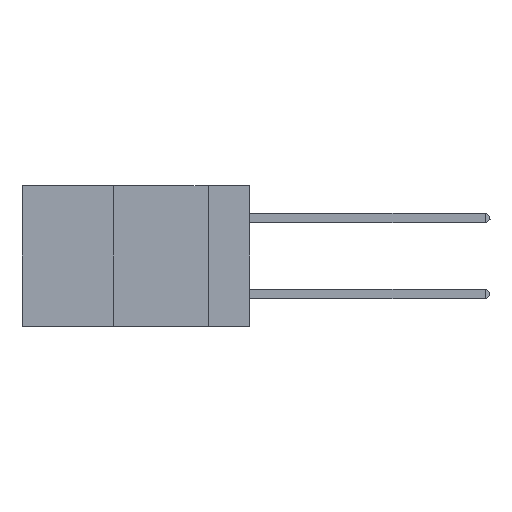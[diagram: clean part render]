
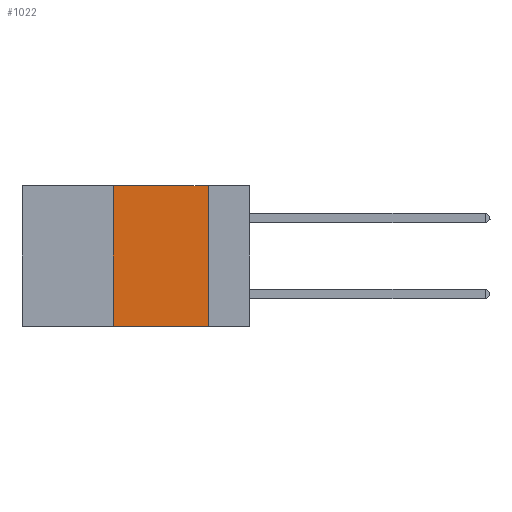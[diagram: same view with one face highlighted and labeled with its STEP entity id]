
A CAD part, left-side view. The second image highlights one B-rep face of the part: STEP entity #1022.
In plain terms, the highlighted planar face has unit normal (-1, 0, 0).
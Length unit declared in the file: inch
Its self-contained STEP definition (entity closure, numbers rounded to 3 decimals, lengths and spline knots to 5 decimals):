
#85 = VERTEX_POINT ( 'NONE', #12212 ) ;
#487 = VERTEX_POINT ( 'NONE', #937 ) ;
#614 = LINE ( 'NONE', #9621, #9235 ) ;
#774 = LINE ( 'NONE', #10442, #9761 ) ;
#937 = CARTESIAN_POINT ( 'NONE',  ( 0., 0.36, 0. ) ) ;
#940 = ORIENTED_EDGE ( 'NONE', *, *, #3587, .F. ) ;
#1022 = ADVANCED_FACE ( 'NONE', ( #4498 ), #13540, .F. ) ;
#1138 = EDGE_LOOP ( 'NONE', ( #940, #3917, #8635, #14436 ) ) ;
#1966 = CARTESIAN_POINT ( 'NONE',  ( 0., 0.36, 0. ) ) ;
#2500 = CARTESIAN_POINT ( 'NONE',  ( 0., 0.11, 0. ) ) ;
#3080 = DIRECTION ( 'NONE',  ( 0., -1., 0. ) ) ;
#3549 = CARTESIAN_POINT ( 'NONE',  ( 0., 0.6, 0. ) ) ;
#3587 = EDGE_CURVE ( 'NONE', #4354, #5332, #614, .T. ) ;
#3619 = DIRECTION ( 'NONE',  ( 0., 0., -1. ) ) ;
#3917 = ORIENTED_EDGE ( 'NONE', *, *, #14448, .F. ) ;
#4169 = AXIS2_PLACEMENT_3D ( 'NONE', #3549, #12437, #3619 ) ;
#4195 = LINE ( 'NONE', #8719, #12751 ) ;
#4354 = VERTEX_POINT ( 'NONE', #2500 ) ;
#4498 = FACE_OUTER_BOUND ( 'NONE', #1138, .T. ) ;
#4576 = DIRECTION ( 'NONE',  ( 0., -1., 0. ) ) ;
#5332 = VERTEX_POINT ( 'NONE', #11375 ) ;
#6788 = LINE ( 'NONE', #1966, #13392 ) ;
#6948 = EDGE_CURVE ( 'NONE', #85, #5332, #774, .T. ) ;
#8635 = ORIENTED_EDGE ( 'NONE', *, *, #12779, .F. ) ;
#8719 = CARTESIAN_POINT ( 'NONE',  ( 0., 0.6, 0. ) ) ;
#9235 = VECTOR ( 'NONE', #14136, 39.37008 ) ;
#9621 = CARTESIAN_POINT ( 'NONE',  ( 0., 0.11, 0. ) ) ;
#9761 = VECTOR ( 'NONE', #4576, 39.37008 ) ;
#10442 = CARTESIAN_POINT ( 'NONE',  ( 0., 0.6, -0.37 ) ) ;
#11375 = CARTESIAN_POINT ( 'NONE',  ( 0., 0.11, -0.37 ) ) ;
#12212 = CARTESIAN_POINT ( 'NONE',  ( 0., 0.36, -0.37 ) ) ;
#12437 = DIRECTION ( 'NONE',  ( 1., 0., 0. ) ) ;
#12751 = VECTOR ( 'NONE', #3080, 39.37008 ) ;
#12779 = EDGE_CURVE ( 'NONE', #85, #487, #6788, .T. ) ;
#13392 = VECTOR ( 'NONE', #14659, 39.37008 ) ;
#13540 = PLANE ( 'NONE',  #4169 ) ;
#14136 = DIRECTION ( 'NONE',  ( 0., 0., -1. ) ) ;
#14436 = ORIENTED_EDGE ( 'NONE', *, *, #6948, .T. ) ;
#14448 = EDGE_CURVE ( 'NONE', #487, #4354, #4195, .T. ) ;
#14659 = DIRECTION ( 'NONE',  ( 0., 0., 1. ) ) ;
